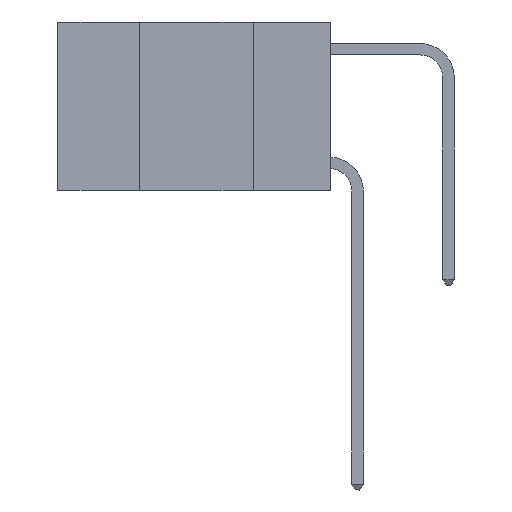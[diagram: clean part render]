
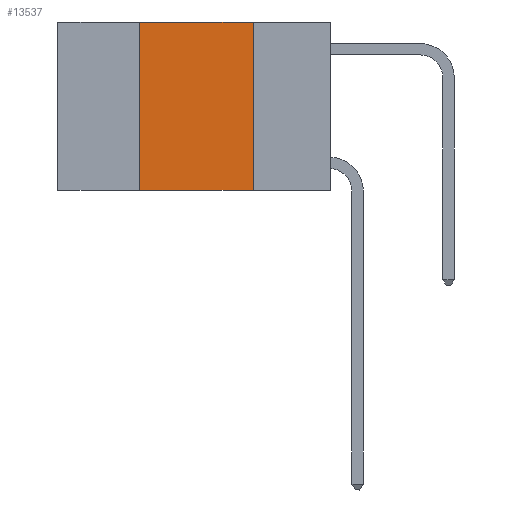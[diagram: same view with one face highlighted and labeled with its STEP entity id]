
A CAD part, left-side view. The second image highlights one B-rep face of the part: STEP entity #13537.
In plain terms, the highlighted planar face has unit normal (-1, 0, 0).
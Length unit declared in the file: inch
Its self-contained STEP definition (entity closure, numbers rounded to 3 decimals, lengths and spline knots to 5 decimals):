
#191 = DIRECTION ( 'NONE',  ( 0., -1., 0. ) ) ;
#584 = ORIENTED_EDGE ( 'NONE', *, *, #4741, .F. ) ;
#1113 = CARTESIAN_POINT ( 'NONE',  ( 0., 0.17, 0. ) ) ;
#1650 = CARTESIAN_POINT ( 'NONE',  ( 0., 0.6, 0. ) ) ;
#2117 = ORIENTED_EDGE ( 'NONE', *, *, #21427, .T. ) ;
#3311 = ORIENTED_EDGE ( 'NONE', *, *, #25522, .F. ) ;
#3732 = FACE_OUTER_BOUND ( 'NONE', #4239, .T. ) ;
#4239 = EDGE_LOOP ( 'NONE', ( #6226, #584, #3311, #2117 ) ) ;
#4480 = VERTEX_POINT ( 'NONE', #11604 ) ;
#4741 = EDGE_CURVE ( 'NONE', #9031, #26328, #24991, .T. ) ;
#5186 = DIRECTION ( 'NONE',  ( 0., -1., 0. ) ) ;
#5835 = DIRECTION ( 'NONE',  ( 1., 0., 0. ) ) ;
#6226 = ORIENTED_EDGE ( 'NONE', *, *, #11208, .F. ) ;
#8717 = VECTOR ( 'NONE', #191, 39.37008 ) ;
#8725 = CARTESIAN_POINT ( 'NONE',  ( 0., 0.42, 0. ) ) ;
#8871 = DIRECTION ( 'NONE',  ( 0., 0., -1. ) ) ;
#9031 = VERTEX_POINT ( 'NONE', #14652 ) ;
#9843 = CARTESIAN_POINT ( 'NONE',  ( 0., 0.17, -0.37 ) ) ;
#9886 = VECTOR ( 'NONE', #5186, 39.37008 ) ;
#11208 = EDGE_CURVE ( 'NONE', #26328, #19915, #19449, .T. ) ;
#11604 = CARTESIAN_POINT ( 'NONE',  ( 0., 0.42, -0.37 ) ) ;
#13537 = ADVANCED_FACE ( 'NONE', ( #3732 ), #13829, .F. ) ;
#13829 = PLANE ( 'NONE',  #24861 ) ;
#14652 = CARTESIAN_POINT ( 'NONE',  ( 0., 0.42, 0. ) ) ;
#15893 = LINE ( 'NONE', #8725, #26121 ) ;
#16404 = CARTESIAN_POINT ( 'NONE',  ( 0., 0.6, 0. ) ) ;
#17357 = CARTESIAN_POINT ( 'NONE',  ( 0., 0.6, -0.37 ) ) ;
#18812 = VECTOR ( 'NONE', #8871, 39.37008 ) ;
#19449 = LINE ( 'NONE', #21078, #18812 ) ;
#19915 = VERTEX_POINT ( 'NONE', #9843 ) ;
#20067 = DIRECTION ( 'NONE',  ( 0., 0., -1. ) ) ;
#20924 = DIRECTION ( 'NONE',  ( 0., 0., 1. ) ) ;
#21078 = CARTESIAN_POINT ( 'NONE',  ( 0., 0.17, 0. ) ) ;
#21427 = EDGE_CURVE ( 'NONE', #4480, #19915, #26137, .T. ) ;
#24861 = AXIS2_PLACEMENT_3D ( 'NONE', #1650, #5835, #20067 ) ;
#24991 = LINE ( 'NONE', #16404, #8717 ) ;
#25522 = EDGE_CURVE ( 'NONE', #4480, #9031, #15893, .T. ) ;
#26121 = VECTOR ( 'NONE', #20924, 39.37008 ) ;
#26137 = LINE ( 'NONE', #17357, #9886 ) ;
#26328 = VERTEX_POINT ( 'NONE', #1113 ) ;
